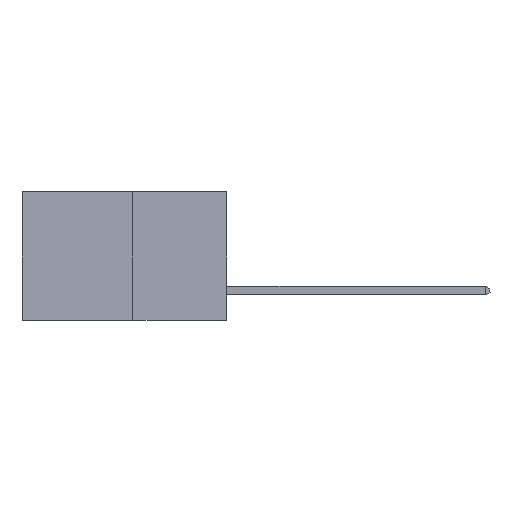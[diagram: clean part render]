
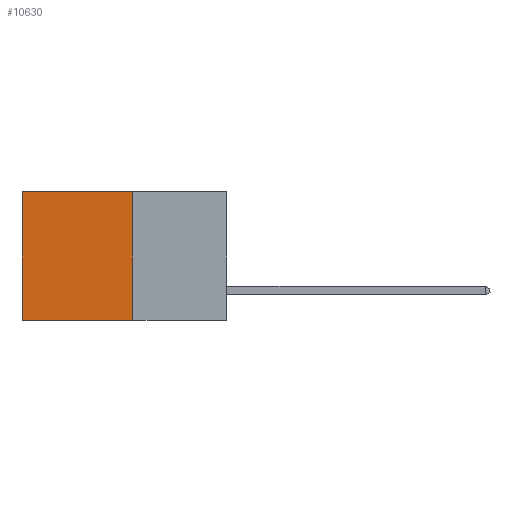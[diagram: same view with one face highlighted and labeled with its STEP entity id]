
A CAD part, left-side view. The second image highlights one B-rep face of the part: STEP entity #10630.
In plain terms, the highlighted planar face has unit normal (-1, 0, 0).
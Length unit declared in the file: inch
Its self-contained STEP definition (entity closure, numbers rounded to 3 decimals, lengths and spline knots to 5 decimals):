
#4 = CARTESIAN_POINT ( 'NONE',  ( 0.277, 0.59, 0. ) ) ;
#299 = EDGE_CURVE ( 'NONE', #11127, #12609, #12060, .T. ) ;
#429 = CARTESIAN_POINT ( 'NONE',  ( 0.277, 0.27, 0. ) ) ;
#1669 = CARTESIAN_POINT ( 'NONE',  ( 0.277, 0.27, -0.37 ) ) ;
#2145 = CARTESIAN_POINT ( 'NONE',  ( 0.277, 0.59, -0.37 ) ) ;
#2619 = PLANE ( 'NONE',  #8710 ) ;
#2724 = DIRECTION ( 'NONE',  ( 0., 0., -1. ) ) ;
#4219 = VERTEX_POINT ( 'NONE', #8227 ) ;
#4631 = DIRECTION ( 'NONE',  ( 1., 0., 0. ) ) ;
#4729 = EDGE_CURVE ( 'NONE', #12609, #4219, #7600, .T. ) ;
#5156 = LINE ( 'NONE', #429, #9198 ) ;
#5223 = EDGE_CURVE ( 'NONE', #5852, #4219, #11854, .T. ) ;
#5266 = ORIENTED_EDGE ( 'NONE', *, *, #10615, .T. ) ;
#5852 = VERTEX_POINT ( 'NONE', #4 ) ;
#6320 = DIRECTION ( 'NONE',  ( 0., 1., 0. ) ) ;
#6523 = VECTOR ( 'NONE', #7894, 39.37008 ) ;
#6537 = FACE_OUTER_BOUND ( 'NONE', #8871, .T. ) ;
#6593 = CARTESIAN_POINT ( 'NONE',  ( 0.277, 0.27, -0.37 ) ) ;
#7558 = DIRECTION ( 'NONE',  ( 0., 1., 0. ) ) ;
#7600 = LINE ( 'NONE', #6593, #12444 ) ;
#7623 = ORIENTED_EDGE ( 'NONE', *, *, #4729, .F. ) ;
#7825 = CARTESIAN_POINT ( 'NONE',  ( 0.277, 0.27, -0.37 ) ) ;
#7894 = DIRECTION ( 'NONE',  ( 0., 0., -1. ) ) ;
#8227 = CARTESIAN_POINT ( 'NONE',  ( 0.277, 0.59, -0.37 ) ) ;
#8710 = AXIS2_PLACEMENT_3D ( 'NONE', #12413, #4631, #11518 ) ;
#8871 = EDGE_LOOP ( 'NONE', ( #9914, #7623, #10223, #5266 ) ) ;
#9198 = VECTOR ( 'NONE', #7558, 39.37008 ) ;
#9914 = ORIENTED_EDGE ( 'NONE', *, *, #5223, .T. ) ;
#10223 = ORIENTED_EDGE ( 'NONE', *, *, #299, .F. ) ;
#10615 = EDGE_CURVE ( 'NONE', #11127, #5852, #5156, .T. ) ;
#10630 = ADVANCED_FACE ( 'NONE', ( #6537 ), #2619, .F. ) ;
#11127 = VERTEX_POINT ( 'NONE', #12165 ) ;
#11518 = DIRECTION ( 'NONE',  ( 0., 0., -1. ) ) ;
#11545 = VECTOR ( 'NONE', #2724, 39.37008 ) ;
#11854 = LINE ( 'NONE', #2145, #11545 ) ;
#12060 = LINE ( 'NONE', #7825, #6523 ) ;
#12165 = CARTESIAN_POINT ( 'NONE',  ( 0.277, 0.27, 0. ) ) ;
#12413 = CARTESIAN_POINT ( 'NONE',  ( 0.277, 0.27, -0.37 ) ) ;
#12444 = VECTOR ( 'NONE', #6320, 39.37008 ) ;
#12609 = VERTEX_POINT ( 'NONE', #1669 ) ;
